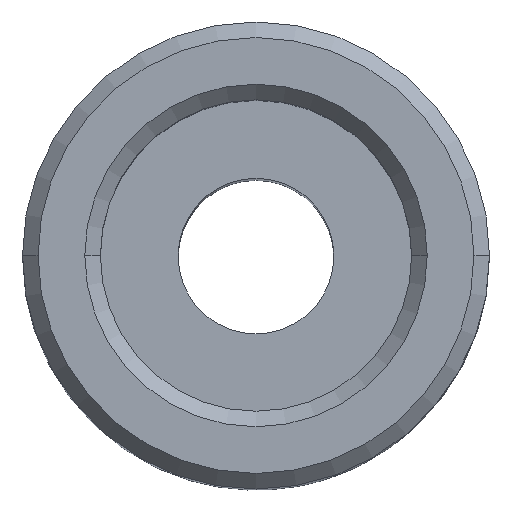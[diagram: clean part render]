
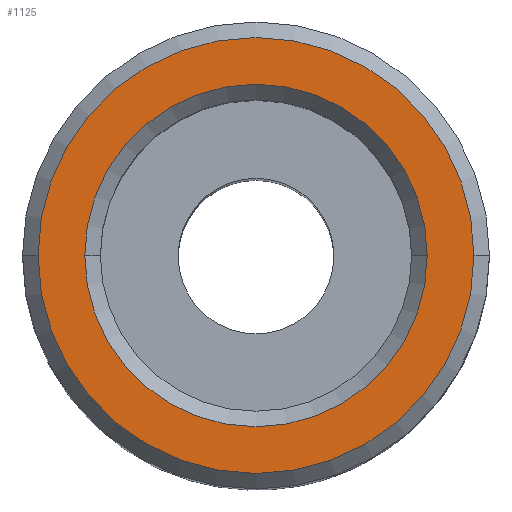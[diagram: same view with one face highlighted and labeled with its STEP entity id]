
A CAD part, top view. The second image highlights one B-rep face of the part: STEP entity #1125.
In plain terms, the highlighted planar face has unit normal (0, 0, 1).
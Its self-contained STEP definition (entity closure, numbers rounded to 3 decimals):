
#21 = CIRCLE ( 'NONE', #1127, 5.5 ) ;
#36 = VERTEX_POINT ( 'NONE', #1192 ) ;
#41 = DIRECTION ( 'NONE',  ( 0., 0., -1. ) ) ;
#48 = DIRECTION ( 'NONE',  ( 1., 0., 0. ) ) ;
#103 = PLANE ( 'NONE',  #634 ) ;
#232 = CARTESIAN_POINT ( 'NONE',  ( -7., 0., 25. ) ) ;
#237 = DIRECTION ( 'NONE',  ( 0., 0., -1. ) ) ;
#247 = AXIS2_PLACEMENT_3D ( 'NONE', #326, #237, #1030 ) ;
#292 = FACE_BOUND ( 'NONE', #593, .T. ) ;
#326 = CARTESIAN_POINT ( 'NONE',  ( 0., 0., 25. ) ) ;
#338 = VERTEX_POINT ( 'NONE', #640 ) ;
#364 = ORIENTED_EDGE ( 'NONE', *, *, #639, .T. ) ;
#402 = CARTESIAN_POINT ( 'NONE',  ( 0., 0., 25. ) ) ;
#455 = DIRECTION ( 'NONE',  ( 0., 0., 1. ) ) ;
#537 = DIRECTION ( 'NONE',  ( 1., 0., 0. ) ) ;
#543 = CARTESIAN_POINT ( 'NONE',  ( 7., 0., 25. ) ) ;
#555 = VERTEX_POINT ( 'NONE', #543 ) ;
#591 = ORIENTED_EDGE ( 'NONE', *, *, #1217, .T. ) ;
#593 = EDGE_LOOP ( 'NONE', ( #591, #661 ) ) ;
#634 = AXIS2_PLACEMENT_3D ( 'NONE', #402, #792, #1183 ) ;
#639 = EDGE_CURVE ( 'NONE', #851, #555, #1008, .T. ) ;
#640 = CARTESIAN_POINT ( 'NONE',  ( -5.5, 0., 25. ) ) ;
#661 = ORIENTED_EDGE ( 'NONE', *, *, #1147, .T. ) ;
#792 = DIRECTION ( 'NONE',  ( 0., 0., 1. ) ) ;
#798 = AXIS2_PLACEMENT_3D ( 'NONE', #800, #1002, #1107 ) ;
#800 = CARTESIAN_POINT ( 'NONE',  ( 0., 0., 25. ) ) ;
#851 = VERTEX_POINT ( 'NONE', #232 ) ;
#863 = CIRCLE ( 'NONE', #798, 7. ) ;
#907 = ORIENTED_EDGE ( 'NONE', *, *, #1171, .T. ) ;
#982 = FACE_OUTER_BOUND ( 'NONE', #1136, .T. ) ;
#1002 = DIRECTION ( 'NONE',  ( 0., 0., 1. ) ) ;
#1008 = CIRCLE ( 'NONE', #1167, 7. ) ;
#1027 = CARTESIAN_POINT ( 'NONE',  ( 0., 0., 25. ) ) ;
#1030 = DIRECTION ( 'NONE',  ( 1., 0., 0. ) ) ;
#1107 = DIRECTION ( 'NONE',  ( 1., 0., 0. ) ) ;
#1125 = ADVANCED_FACE ( 'NONE', ( #292, #982 ), #103, .T. ) ;
#1127 = AXIS2_PLACEMENT_3D ( 'NONE', #1197, #41, #48 ) ;
#1136 = EDGE_LOOP ( 'NONE', ( #364, #907 ) ) ;
#1147 = EDGE_CURVE ( 'NONE', #338, #36, #21, .T. ) ;
#1166 = CIRCLE ( 'NONE', #247, 5.5 ) ;
#1167 = AXIS2_PLACEMENT_3D ( 'NONE', #1027, #455, #537 ) ;
#1171 = EDGE_CURVE ( 'NONE', #555, #851, #863, .T. ) ;
#1183 = DIRECTION ( 'NONE',  ( 1., 0., 0. ) ) ;
#1192 = CARTESIAN_POINT ( 'NONE',  ( 5.5, 0., 25. ) ) ;
#1197 = CARTESIAN_POINT ( 'NONE',  ( 0., 0., 25. ) ) ;
#1217 = EDGE_CURVE ( 'NONE', #36, #338, #1166, .T. ) ;
